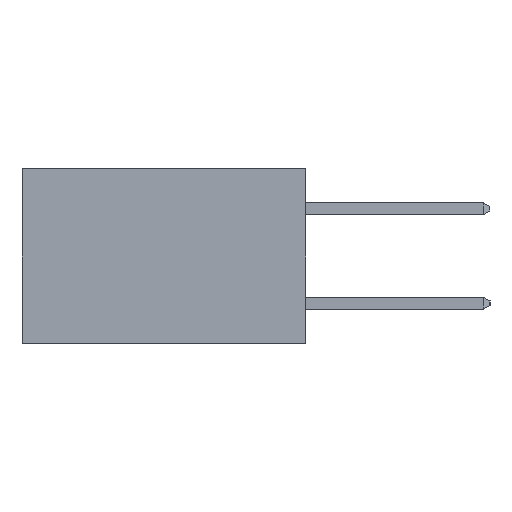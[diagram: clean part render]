
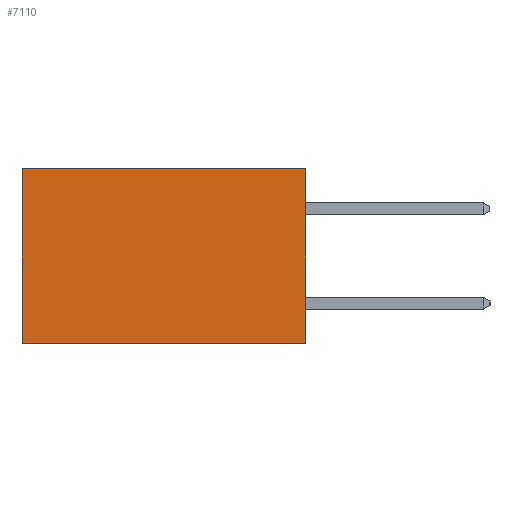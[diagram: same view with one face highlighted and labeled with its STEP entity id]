
A CAD part, left-side view. The second image highlights one B-rep face of the part: STEP entity #7110.
In plain terms, the highlighted planar face has unit normal (-1, 0, 0).
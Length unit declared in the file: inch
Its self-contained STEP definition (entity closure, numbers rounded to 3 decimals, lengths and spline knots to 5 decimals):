
#188 = FACE_OUTER_BOUND ( 'NONE', #8323, .T. ) ;
#442 = VERTEX_POINT ( 'NONE', #3286 ) ;
#800 = VECTOR ( 'NONE', #12812, 39.37008 ) ;
#1327 = VECTOR ( 'NONE', #8600, 39.37008 ) ;
#2061 = DIRECTION ( 'NONE',  ( 0., 0., -1. ) ) ;
#2113 = PLANE ( 'NONE',  #3106 ) ;
#2230 = CARTESIAN_POINT ( 'NONE',  ( 0.2615, 0., -0.37 ) ) ;
#2315 = DIRECTION ( 'NONE',  ( 1., 0., 0. ) ) ;
#2427 = CARTESIAN_POINT ( 'NONE',  ( 0.2615, 0., 0. ) ) ;
#3085 = LINE ( 'NONE', #7827, #800 ) ;
#3106 = AXIS2_PLACEMENT_3D ( 'NONE', #2230, #2315, #2061 ) ;
#3286 = CARTESIAN_POINT ( 'NONE',  ( 0.2615, 0.6, -0.37 ) ) ;
#3581 = LINE ( 'NONE', #9861, #1327 ) ;
#4099 = CARTESIAN_POINT ( 'NONE',  ( 0.2615, 0.6, 0. ) ) ;
#5512 = EDGE_CURVE ( 'NONE', #10045, #7784, #3581, .T. ) ;
#6807 = DIRECTION ( 'NONE',  ( 0., 1., 0. ) ) ;
#7110 = ADVANCED_FACE ( 'NONE', ( #188 ), #2113, .F. ) ;
#7356 = VERTEX_POINT ( 'NONE', #4099 ) ;
#7465 = LINE ( 'NONE', #8717, #12510 ) ;
#7717 = LINE ( 'NONE', #11485, #10861 ) ;
#7784 = VERTEX_POINT ( 'NONE', #9414 ) ;
#7827 = CARTESIAN_POINT ( 'NONE',  ( 0.2615, 0.6, -0.37 ) ) ;
#8323 = EDGE_LOOP ( 'NONE', ( #11262, #11393, #11276, #10244 ) ) ;
#8600 = DIRECTION ( 'NONE',  ( 0., 0., -1. ) ) ;
#8717 = CARTESIAN_POINT ( 'NONE',  ( 0.2615, 0., -0.37 ) ) ;
#8987 = EDGE_CURVE ( 'NONE', #7784, #442, #7465, .T. ) ;
#9414 = CARTESIAN_POINT ( 'NONE',  ( 0.2615, 0., -0.37 ) ) ;
#9861 = CARTESIAN_POINT ( 'NONE',  ( 0.2615, 0., -0.37 ) ) ;
#10045 = VERTEX_POINT ( 'NONE', #2427 ) ;
#10244 = ORIENTED_EDGE ( 'NONE', *, *, #10758, .T. ) ;
#10758 = EDGE_CURVE ( 'NONE', #10045, #7356, #7717, .T. ) ;
#10861 = VECTOR ( 'NONE', #11528, 39.37008 ) ;
#11262 = ORIENTED_EDGE ( 'NONE', *, *, #12525, .T. ) ;
#11276 = ORIENTED_EDGE ( 'NONE', *, *, #5512, .F. ) ;
#11393 = ORIENTED_EDGE ( 'NONE', *, *, #8987, .F. ) ;
#11485 = CARTESIAN_POINT ( 'NONE',  ( 0.2615, 0., 0. ) ) ;
#11528 = DIRECTION ( 'NONE',  ( 0., 1., 0. ) ) ;
#12510 = VECTOR ( 'NONE', #6807, 39.37008 ) ;
#12525 = EDGE_CURVE ( 'NONE', #7356, #442, #3085, .T. ) ;
#12812 = DIRECTION ( 'NONE',  ( 0., 0., -1. ) ) ;
